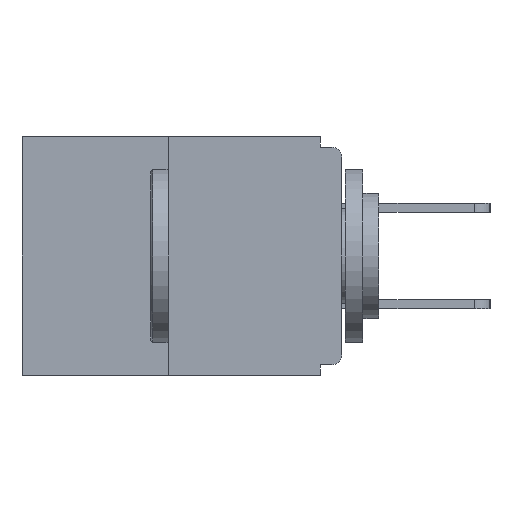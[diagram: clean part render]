
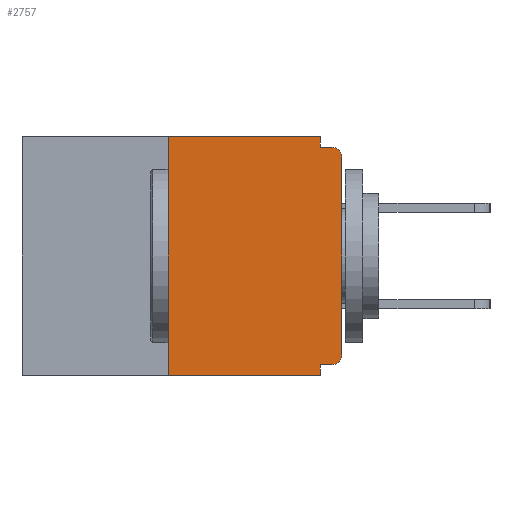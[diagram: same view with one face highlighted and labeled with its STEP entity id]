
A CAD part, left-side view. The second image highlights one B-rep face of the part: STEP entity #2757.
In plain terms, the highlighted planar face has unit normal (-1, 0, 0).
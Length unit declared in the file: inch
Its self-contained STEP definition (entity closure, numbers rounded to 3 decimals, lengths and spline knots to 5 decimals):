
#240 = VERTEX_POINT ( 'NONE', #18037 ) ;
#536 = DIRECTION ( 'NONE',  ( 0., 0., 1. ) ) ;
#671 = LINE ( 'NONE', #27263, #23134 ) ;
#1053 = VERTEX_POINT ( 'NONE', #22113 ) ;
#1398 = CARTESIAN_POINT ( 'NONE',  ( 0., 0., 0. ) ) ;
#1513 = DIRECTION ( 'NONE',  ( 0., 1., 0. ) ) ;
#1682 = VECTOR ( 'NONE', #3813, 39.37008 ) ;
#1799 = DIRECTION ( 'NONE',  ( 0., 0., -1. ) ) ;
#1987 = CARTESIAN_POINT ( 'NONE',  ( 0., 0.015, -0.328 ) ) ;
#2553 = DIRECTION ( 'NONE',  ( 1., 0., 0. ) ) ;
#2757 = ADVANCED_FACE ( 'NONE', ( #9197 ), #24924, .F. ) ;
#3175 = CARTESIAN_POINT ( 'NONE',  ( 0., 0.46, 0. ) ) ;
#3563 = VECTOR ( 'NONE', #536, 39.37008 ) ;
#3813 = DIRECTION ( 'NONE',  ( 0., 0., -1. ) ) ;
#4395 = CARTESIAN_POINT ( 'NONE',  ( 0., 0.015, -0.313 ) ) ;
#4792 = DIRECTION ( 'NONE',  ( 0., 0., -1. ) ) ;
#5513 = DIRECTION ( 'NONE',  ( 0., -1., 0. ) ) ;
#6244 = ORIENTED_EDGE ( 'NONE', *, *, #17623, .T. ) ;
#6669 = VECTOR ( 'NONE', #1513, 39.37008 ) ;
#6751 = AXIS2_PLACEMENT_3D ( 'NONE', #4395, #20094, #11143 ) ;
#6981 = VECTOR ( 'NONE', #26866, 39.37008 ) ;
#7136 = VERTEX_POINT ( 'NONE', #1987 ) ;
#7361 = CARTESIAN_POINT ( 'NONE',  ( 0., 0.25, 0. ) ) ;
#8130 = CARTESIAN_POINT ( 'NONE',  ( 0., 0.031, -0.015 ) ) ;
#8696 = LINE ( 'NONE', #23215, #21379 ) ;
#8745 = CARTESIAN_POINT ( 'NONE',  ( 0., 0., -0.313 ) ) ;
#8803 = DIRECTION ( 'NONE',  ( 0., 0., 1. ) ) ;
#9024 = ORIENTED_EDGE ( 'NONE', *, *, #9987, .F. ) ;
#9028 = DIRECTION ( 'NONE',  ( 0., -1., 0. ) ) ;
#9197 = FACE_OUTER_BOUND ( 'NONE', #27937, .T. ) ;
#9458 = CIRCLE ( 'NONE', #6751, 0.015 ) ;
#9900 = EDGE_CURVE ( 'NONE', #1053, #14028, #671, .T. ) ;
#9987 = EDGE_CURVE ( 'NONE', #16882, #14028, #8696, .T. ) ;
#10323 = ORIENTED_EDGE ( 'NONE', *, *, #22581, .T. ) ;
#11143 = DIRECTION ( 'NONE',  ( 0., 0., -1. ) ) ;
#11448 = CARTESIAN_POINT ( 'NONE',  ( 0., 0.46, 0. ) ) ;
#11471 = VERTEX_POINT ( 'NONE', #8745 ) ;
#11658 = AXIS2_PLACEMENT_3D ( 'NONE', #24575, #22180, #1799 ) ;
#12577 = ORIENTED_EDGE ( 'NONE', *, *, #26008, .F. ) ;
#12633 = LINE ( 'NONE', #19447, #6669 ) ;
#14028 = VERTEX_POINT ( 'NONE', #16425 ) ;
#14496 = VECTOR ( 'NONE', #8803, 39.37008 ) ;
#16382 = EDGE_CURVE ( 'NONE', #1053, #18880, #27863, .T. ) ;
#16425 = CARTESIAN_POINT ( 'NONE',  ( 0., 0.031, -0.343 ) ) ;
#16594 = ORIENTED_EDGE ( 'NONE', *, *, #18715, .T. ) ;
#16728 = CARTESIAN_POINT ( 'NONE',  ( 0., 0.031, -0.328 ) ) ;
#16877 = VERTEX_POINT ( 'NONE', #18879 ) ;
#16882 = VERTEX_POINT ( 'NONE', #16728 ) ;
#17423 = ORIENTED_EDGE ( 'NONE', *, *, #16382, .F. ) ;
#17623 = EDGE_CURVE ( 'NONE', #7136, #11471, #9458, .T. ) ;
#17756 = AXIS2_PLACEMENT_3D ( 'NONE', #11448, #2553, #4792 ) ;
#18037 = CARTESIAN_POINT ( 'NONE',  ( 0., 0.031, 0. ) ) ;
#18322 = EDGE_CURVE ( 'NONE', #21240, #18893, #22078, .T. ) ;
#18715 = EDGE_CURVE ( 'NONE', #16877, #18893, #19592, .T. ) ;
#18879 = CARTESIAN_POINT ( 'NONE',  ( 0., 0., -0.03 ) ) ;
#18880 = VERTEX_POINT ( 'NONE', #26401 ) ;
#18893 = VERTEX_POINT ( 'NONE', #21961 ) ;
#19447 = CARTESIAN_POINT ( 'NONE',  ( 0., 0., -0.328 ) ) ;
#19592 = CIRCLE ( 'NONE', #11658, 0.015 ) ;
#20094 = DIRECTION ( 'NONE',  ( -1., 0., 0. ) ) ;
#20460 = VECTOR ( 'NONE', #5513, 39.37008 ) ;
#20472 = ORIENTED_EDGE ( 'NONE', *, *, #27050, .F. ) ;
#21240 = VERTEX_POINT ( 'NONE', #8130 ) ;
#21379 = VECTOR ( 'NONE', #25480, 39.37008 ) ;
#21872 = LINE ( 'NONE', #1398, #14496 ) ;
#21961 = CARTESIAN_POINT ( 'NONE',  ( 0., 0.015, -0.015 ) ) ;
#22078 = LINE ( 'NONE', #22703, #6981 ) ;
#22113 = CARTESIAN_POINT ( 'NONE',  ( 0., 0.25, -0.343 ) ) ;
#22180 = DIRECTION ( 'NONE',  ( -1., 0., 0. ) ) ;
#22581 = EDGE_CURVE ( 'NONE', #11471, #16877, #21872, .T. ) ;
#22703 = CARTESIAN_POINT ( 'NONE',  ( 0., 0., -0.015 ) ) ;
#23134 = VECTOR ( 'NONE', #9028, 39.37008 ) ;
#23215 = CARTESIAN_POINT ( 'NONE',  ( 0., 0.031, -0.343 ) ) ;
#23272 = ORIENTED_EDGE ( 'NONE', *, *, #9900, .T. ) ;
#23476 = ORIENTED_EDGE ( 'NONE', *, *, #23593, .F. ) ;
#23593 = EDGE_CURVE ( 'NONE', #240, #21240, #24531, .T. ) ;
#24465 = ORIENTED_EDGE ( 'NONE', *, *, #18322, .F. ) ;
#24531 = LINE ( 'NONE', #28107, #1682 ) ;
#24575 = CARTESIAN_POINT ( 'NONE',  ( 0., 0.015, -0.03 ) ) ;
#24924 = PLANE ( 'NONE',  #17756 ) ;
#25480 = DIRECTION ( 'NONE',  ( 0., 0., -1. ) ) ;
#26008 = EDGE_CURVE ( 'NONE', #18880, #240, #26079, .T. ) ;
#26079 = LINE ( 'NONE', #3175, #20460 ) ;
#26401 = CARTESIAN_POINT ( 'NONE',  ( 0., 0.25, 0. ) ) ;
#26866 = DIRECTION ( 'NONE',  ( 0., -1., 0. ) ) ;
#27050 = EDGE_CURVE ( 'NONE', #7136, #16882, #12633, .T. ) ;
#27263 = CARTESIAN_POINT ( 'NONE',  ( 0., 0.46, -0.343 ) ) ;
#27863 = LINE ( 'NONE', #7361, #3563 ) ;
#27937 = EDGE_LOOP ( 'NONE', ( #12577, #17423, #23272, #9024, #20472, #6244, #10323, #16594, #24465, #23476 ) ) ;
#28107 = CARTESIAN_POINT ( 'NONE',  ( 0., 0.031, 0. ) ) ;
